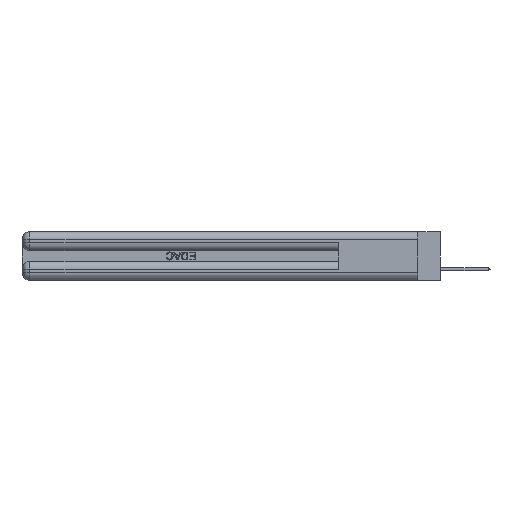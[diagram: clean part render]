
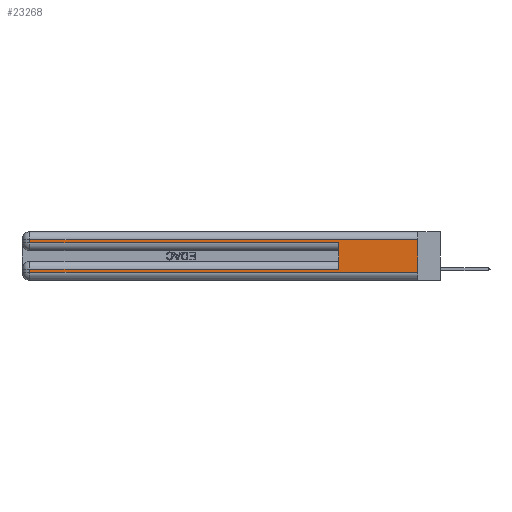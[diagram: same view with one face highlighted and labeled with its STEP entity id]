
A CAD part, left-side view. The second image highlights one B-rep face of the part: STEP entity #23268.
In plain terms, the highlighted planar face has unit normal (-1, 0, 0).
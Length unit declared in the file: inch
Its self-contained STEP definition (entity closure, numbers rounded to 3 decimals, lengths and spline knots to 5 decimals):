
#1773 = ORIENTED_EDGE ( 'NONE', *, *, #23262, .T. ) ;
#3401 = DIRECTION ( 'NONE',  ( 0., 0., -1. ) ) ;
#4675 = EDGE_CURVE ( 'NONE', #43517, #12546, #37398, .T. ) ;
#4976 = VERTEX_POINT ( 'NONE', #20112 ) ;
#5219 = DIRECTION ( 'NONE',  ( 0., 0., -1. ) ) ;
#5717 = CARTESIAN_POINT ( 'NONE',  ( 0., 2.94, 0.06 ) ) ;
#5820 = FACE_OUTER_BOUND ( 'NONE', #25505, .T. ) ;
#7093 = LINE ( 'NONE', #36601, #16046 ) ;
#7394 = VECTOR ( 'NONE', #3401, 39.37008 ) ;
#7788 = VECTOR ( 'NONE', #35221, 39.37008 ) ;
#9152 = LINE ( 'NONE', #29189, #36318 ) ;
#9732 = ORIENTED_EDGE ( 'NONE', *, *, #49557, .F. ) ;
#10469 = EDGE_CURVE ( 'NONE', #12546, #22727, #9152, .T. ) ;
#12546 = VERTEX_POINT ( 'NONE', #37020 ) ;
#12696 = ORIENTED_EDGE ( 'NONE', *, *, #30051, .T. ) ;
#14121 = DIRECTION ( 'NONE',  ( 0., 0., -1. ) ) ;
#14241 = CARTESIAN_POINT ( 'NONE',  ( 0., 0.6, 0.285 ) ) ;
#16046 = VECTOR ( 'NONE', #20732, 39.37008 ) ;
#16583 = DIRECTION ( 'NONE',  ( 0., 0., 1. ) ) ;
#17164 = VERTEX_POINT ( 'NONE', #47252 ) ;
#17881 = LINE ( 'NONE', #27983, #20278 ) ;
#19547 = ORIENTED_EDGE ( 'NONE', *, *, #49265, .T. ) ;
#20112 = CARTESIAN_POINT ( 'NONE',  ( 0., 2.94, 0.085 ) ) ;
#20278 = VECTOR ( 'NONE', #39283, 39.37008 ) ;
#20732 = DIRECTION ( 'NONE',  ( 0., 1., 0. ) ) ;
#21010 = LINE ( 'NONE', #24039, #7788 ) ;
#21650 = VERTEX_POINT ( 'NONE', #44236 ) ;
#22113 = VECTOR ( 'NONE', #16583, 39.37008 ) ;
#22727 = VERTEX_POINT ( 'NONE', #14241 ) ;
#23262 = EDGE_CURVE ( 'NONE', #21650, #4976, #7093, .T. ) ;
#23268 = ADVANCED_FACE ( 'NONE', ( #5820 ), #40622, .F. ) ;
#23573 = EDGE_CURVE ( 'NONE', #21650, #22727, #35328, .T. ) ;
#24039 = CARTESIAN_POINT ( 'NONE',  ( 0., 0., 0.37 ) ) ;
#24737 = VECTOR ( 'NONE', #45421, 39.37008 ) ;
#25505 = EDGE_LOOP ( 'NONE', ( #9732, #34198, #33311, #48472, #30851, #1773, #19547, #12696 ) ) ;
#26550 = EDGE_CURVE ( 'NONE', #17164, #43517, #17881, .T. ) ;
#27973 = CARTESIAN_POINT ( 'NONE',  ( 0., 0.6, 0.145 ) ) ;
#27983 = CARTESIAN_POINT ( 'NONE',  ( 0., 0., 0.31 ) ) ;
#29189 = CARTESIAN_POINT ( 'NONE',  ( 0., 0., 0.285 ) ) ;
#30051 = EDGE_CURVE ( 'NONE', #42579, #36962, #37462, .T. ) ;
#30851 = ORIENTED_EDGE ( 'NONE', *, *, #23573, .F. ) ;
#33311 = ORIENTED_EDGE ( 'NONE', *, *, #4675, .T. ) ;
#33314 = LINE ( 'NONE', #37827, #7394 ) ;
#34198 = ORIENTED_EDGE ( 'NONE', *, *, #26550, .T. ) ;
#34848 = CARTESIAN_POINT ( 'NONE',  ( 0., 0., 0.06 ) ) ;
#35221 = DIRECTION ( 'NONE',  ( 0., 0., -1. ) ) ;
#35328 = LINE ( 'NONE', #27973, #22113 ) ;
#36318 = VECTOR ( 'NONE', #48905, 39.37008 ) ;
#36396 = AXIS2_PLACEMENT_3D ( 'NONE', #36764, #43840, #5219 ) ;
#36601 = CARTESIAN_POINT ( 'NONE',  ( 0., 0., 0.085 ) ) ;
#36764 = CARTESIAN_POINT ( 'NONE',  ( 0., 0., 0.37 ) ) ;
#36962 = VERTEX_POINT ( 'NONE', #47470 ) ;
#37020 = CARTESIAN_POINT ( 'NONE',  ( 0., 2.94, 0.285 ) ) ;
#37398 = LINE ( 'NONE', #40948, #47582 ) ;
#37462 = LINE ( 'NONE', #34848, #24737 ) ;
#37827 = CARTESIAN_POINT ( 'NONE',  ( 0., 2.94, 0.37 ) ) ;
#38583 = CARTESIAN_POINT ( 'NONE',  ( 0., 2.94, 0.31 ) ) ;
#39283 = DIRECTION ( 'NONE',  ( 0., 1., 0. ) ) ;
#40622 = PLANE ( 'NONE',  #36396 ) ;
#40948 = CARTESIAN_POINT ( 'NONE',  ( 0., 2.94, 0.37 ) ) ;
#42579 = VERTEX_POINT ( 'NONE', #5717 ) ;
#43517 = VERTEX_POINT ( 'NONE', #38583 ) ;
#43840 = DIRECTION ( 'NONE',  ( 1., 0., 0. ) ) ;
#44236 = CARTESIAN_POINT ( 'NONE',  ( 0., 0.6, 0.085 ) ) ;
#45421 = DIRECTION ( 'NONE',  ( 0., -1., 0. ) ) ;
#47252 = CARTESIAN_POINT ( 'NONE',  ( 0., 0., 0.31 ) ) ;
#47470 = CARTESIAN_POINT ( 'NONE',  ( 0., 0., 0.06 ) ) ;
#47582 = VECTOR ( 'NONE', #14121, 39.37008 ) ;
#48472 = ORIENTED_EDGE ( 'NONE', *, *, #10469, .T. ) ;
#48905 = DIRECTION ( 'NONE',  ( 0., -1., 0. ) ) ;
#49265 = EDGE_CURVE ( 'NONE', #4976, #42579, #33314, .T. ) ;
#49557 = EDGE_CURVE ( 'NONE', #17164, #36962, #21010, .T. ) ;
